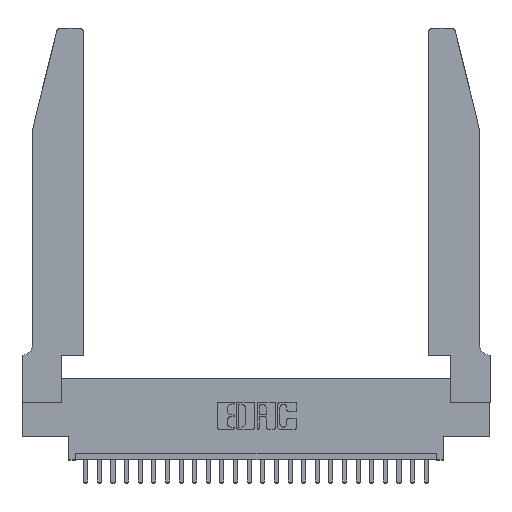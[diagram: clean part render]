
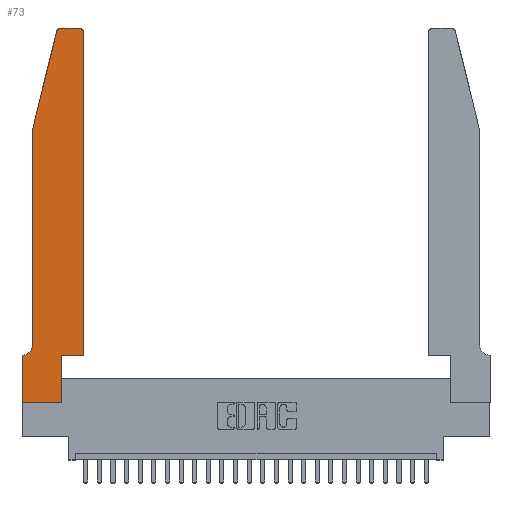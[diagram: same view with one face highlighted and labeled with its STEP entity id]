
A CAD part, top view. The second image highlights one B-rep face of the part: STEP entity #73.
In plain terms, the highlighted planar face has unit normal (0, 0, 1).
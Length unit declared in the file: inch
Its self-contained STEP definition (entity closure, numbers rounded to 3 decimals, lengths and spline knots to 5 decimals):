
#73 = ADVANCED_FACE ( 'NONE', ( #1815 ), #3202, .T. ) ;
#458 = ORIENTED_EDGE ( 'NONE', *, *, #1521, .T. ) ;
#729 = VERTEX_POINT ( 'NONE', #8647 ) ;
#863 = EDGE_CURVE ( 'NONE', #2356, #729, #6350, .T. ) ;
#934 = AXIS2_PLACEMENT_3D ( 'NONE', #18185, #9573, #19917 ) ;
#951 = DIRECTION ( 'NONE',  ( 1., 0., 0. ) ) ;
#974 = DIRECTION ( 'NONE',  ( 0., 1., 0. ) ) ;
#1025 = EDGE_LOOP ( 'NONE', ( #23520, #13581, #13650, #9437, #19073, #15550, #17396, #12224, #4940, #5912, #21403, #458 ) ) ;
#1042 = CARTESIAN_POINT ( 'NONE',  ( 0.25487, 2.72718, 0.37 ) ) ;
#1484 = EDGE_CURVE ( 'NONE', #5299, #7082, #13442, .T. ) ;
#1521 = EDGE_CURVE ( 'NONE', #24458, #5299, #23378, .T. ) ;
#1535 = CARTESIAN_POINT ( 'NONE',  ( 0.0755, 2., 0.37 ) ) ;
#1795 = CARTESIAN_POINT ( 'NONE',  ( 0.2865, 0.35, 0.37 ) ) ;
#1815 = FACE_OUTER_BOUND ( 'NONE', #1025, .T. ) ;
#1866 = CARTESIAN_POINT ( 'NONE',  ( 0.4505, 0.35, 0.37 ) ) ;
#1972 = CARTESIAN_POINT ( 'NONE',  ( 0.0755, 0.35, 0.37 ) ) ;
#2306 = DIRECTION ( 'NONE',  ( -1., 0., 0. ) ) ;
#2356 = VERTEX_POINT ( 'NONE', #11200 ) ;
#2425 = VERTEX_POINT ( 'NONE', #16874 ) ;
#3202 = PLANE ( 'NONE',  #24638 ) ;
#3224 = LINE ( 'NONE', #1866, #24186 ) ;
#3393 = DIRECTION ( 'NONE',  ( 0., -1., 0. ) ) ;
#3413 = LINE ( 'NONE', #4399, #24336 ) ;
#3448 = CARTESIAN_POINT ( 'NONE',  ( 0., 0., 0.37 ) ) ;
#3792 = CARTESIAN_POINT ( 'NONE',  ( 0.0755, 2., 0.37 ) ) ;
#4176 = DIRECTION ( 'NONE',  ( 0., 1., 0. ) ) ;
#4399 = CARTESIAN_POINT ( 'NONE',  ( 0., 0., 0.37 ) ) ;
#4548 = DIRECTION ( 'NONE',  ( -1., 0., 0. ) ) ;
#4625 = VERTEX_POINT ( 'NONE', #7353 ) ;
#4763 = CARTESIAN_POINT ( 'NONE',  ( 0.2865, 0.35, 0.37 ) ) ;
#4940 = ORIENTED_EDGE ( 'NONE', *, *, #15258, .T. ) ;
#5124 = VECTOR ( 'NONE', #3393, 39.37008 ) ;
#5149 = DIRECTION ( 'NONE',  ( 0., 0., 1. ) ) ;
#5299 = VERTEX_POINT ( 'NONE', #26709 ) ;
#5432 = AXIS2_PLACEMENT_3D ( 'NONE', #20993, #10944, #18765 ) ;
#5434 = LINE ( 'NONE', #3792, #8011 ) ;
#5912 = ORIENTED_EDGE ( 'NONE', *, *, #19473, .T. ) ;
#6350 = LINE ( 'NONE', #1972, #11227 ) ;
#6745 = DIRECTION ( 'NONE',  ( 0., -1., 0. ) ) ;
#7082 = VERTEX_POINT ( 'NONE', #20392 ) ;
#7315 = CARTESIAN_POINT ( 'NONE',  ( 0.4505, 2.72, 0.37 ) ) ;
#7353 = CARTESIAN_POINT ( 'NONE',  ( 0.0755, 2., 0.37 ) ) ;
#7660 = VERTEX_POINT ( 'NONE', #3448 ) ;
#7667 = VECTOR ( 'NONE', #974, 39.37008 ) ;
#8011 = VECTOR ( 'NONE', #24451, 39.37008 ) ;
#8265 = DIRECTION ( 'NONE',  ( -1., 0., 0. ) ) ;
#8647 = CARTESIAN_POINT ( 'NONE',  ( 0., 0.35, 0.37 ) ) ;
#8922 = VERTEX_POINT ( 'NONE', #14346 ) ;
#9437 = ORIENTED_EDGE ( 'NONE', *, *, #24647, .T. ) ;
#9573 = DIRECTION ( 'NONE',  ( 0., 0., 1. ) ) ;
#10944 = DIRECTION ( 'NONE',  ( 0., 0., 1. ) ) ;
#11200 = CARTESIAN_POINT ( 'NONE',  ( 0.0055, 0.35, 0.37 ) ) ;
#11216 = LINE ( 'NONE', #1795, #7667 ) ;
#11227 = VECTOR ( 'NONE', #8265, 39.37008 ) ;
#12224 = ORIENTED_EDGE ( 'NONE', *, *, #22583, .T. ) ;
#13150 = VERTEX_POINT ( 'NONE', #4763 ) ;
#13433 = LINE ( 'NONE', #25670, #17614 ) ;
#13442 = LINE ( 'NONE', #22888, #23700 ) ;
#13581 = ORIENTED_EDGE ( 'NONE', *, *, #26428, .T. ) ;
#13650 = ORIENTED_EDGE ( 'NONE', *, *, #17140, .T. ) ;
#13847 = CARTESIAN_POINT ( 'NONE',  ( 0., 0., 0.37 ) ) ;
#14164 = VERTEX_POINT ( 'NONE', #15591 ) ;
#14346 = CARTESIAN_POINT ( 'NONE',  ( 0.4505, 0.35, 0.37 ) ) ;
#14829 = EDGE_CURVE ( 'NONE', #2425, #2356, #24353, .T. ) ;
#15258 = EDGE_CURVE ( 'NONE', #14164, #13150, #11216, .T. ) ;
#15429 = EDGE_CURVE ( 'NONE', #729, #7660, #3413, .T. ) ;
#15550 = ORIENTED_EDGE ( 'NONE', *, *, #863, .T. ) ;
#15591 = CARTESIAN_POINT ( 'NONE',  ( 0.2865, 0., 0.37 ) ) ;
#16487 = AXIS2_PLACEMENT_3D ( 'NONE', #23143, #22260, #2306 ) ;
#16874 = CARTESIAN_POINT ( 'NONE',  ( 0.0755, 0.42, 0.37 ) ) ;
#17140 = EDGE_CURVE ( 'NONE', #22991, #4625, #5434, .T. ) ;
#17263 = CIRCLE ( 'NONE', #5432, 0.03 ) ;
#17396 = ORIENTED_EDGE ( 'NONE', *, *, #15429, .T. ) ;
#17493 = CARTESIAN_POINT ( 'NONE',  ( 0., 0.35, 0.37 ) ) ;
#17614 = VECTOR ( 'NONE', #951, 39.37008 ) ;
#18185 = CARTESIAN_POINT ( 'NONE',  ( 0.4205, 2.72, 0.37 ) ) ;
#18765 = DIRECTION ( 'NONE',  ( 1., 0., 0. ) ) ;
#19073 = ORIENTED_EDGE ( 'NONE', *, *, #14829, .T. ) ;
#19473 = EDGE_CURVE ( 'NONE', #13150, #8922, #13433, .T. ) ;
#19505 = DIRECTION ( 'NONE',  ( 1., 0., 0. ) ) ;
#19917 = DIRECTION ( 'NONE',  ( 1., 0., 0. ) ) ;
#20392 = CARTESIAN_POINT ( 'NONE',  ( 0.284, 2.75, 0.37 ) ) ;
#20993 = CARTESIAN_POINT ( 'NONE',  ( 0.284, 2.72, 0.37 ) ) ;
#21289 = LINE ( 'NONE', #13847, #23820 ) ;
#21403 = ORIENTED_EDGE ( 'NONE', *, *, #22702, .T. ) ;
#21853 = LINE ( 'NONE', #1535, #5124 ) ;
#22260 = DIRECTION ( 'NONE',  ( 0., 0., -1. ) ) ;
#22583 = EDGE_CURVE ( 'NONE', #7660, #14164, #21289, .T. ) ;
#22702 = EDGE_CURVE ( 'NONE', #8922, #24458, #3224, .T. ) ;
#22888 = CARTESIAN_POINT ( 'NONE',  ( 0.2605, 2.75, 0.37 ) ) ;
#22991 = VERTEX_POINT ( 'NONE', #1042 ) ;
#23143 = CARTESIAN_POINT ( 'NONE',  ( 0.0055, 0.42, 0.37 ) ) ;
#23378 = CIRCLE ( 'NONE', #934, 0.03 ) ;
#23520 = ORIENTED_EDGE ( 'NONE', *, *, #1484, .T. ) ;
#23700 = VECTOR ( 'NONE', #4548, 39.37008 ) ;
#23820 = VECTOR ( 'NONE', #23986, 39.37008 ) ;
#23986 = DIRECTION ( 'NONE',  ( 1., 0., 0. ) ) ;
#24186 = VECTOR ( 'NONE', #4176, 39.37008 ) ;
#24336 = VECTOR ( 'NONE', #6745, 39.37008 ) ;
#24353 = CIRCLE ( 'NONE', #16487, 0.07 ) ;
#24451 = DIRECTION ( 'NONE',  ( -0.239, -0.971, 0. ) ) ;
#24458 = VERTEX_POINT ( 'NONE', #7315 ) ;
#24638 = AXIS2_PLACEMENT_3D ( 'NONE', #17493, #5149, #19505 ) ;
#24647 = EDGE_CURVE ( 'NONE', #4625, #2425, #21853, .T. ) ;
#25670 = CARTESIAN_POINT ( 'NONE',  ( 0.4505, 0.35, 0.37 ) ) ;
#26428 = EDGE_CURVE ( 'NONE', #7082, #22991, #17263, .T. ) ;
#26709 = CARTESIAN_POINT ( 'NONE',  ( 0.4205, 2.75, 0.37 ) ) ;
